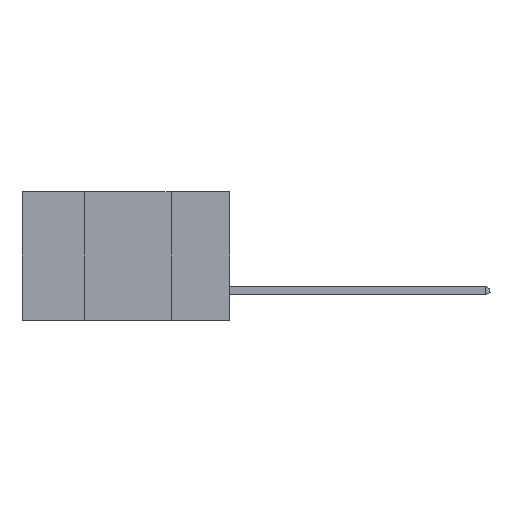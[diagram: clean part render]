
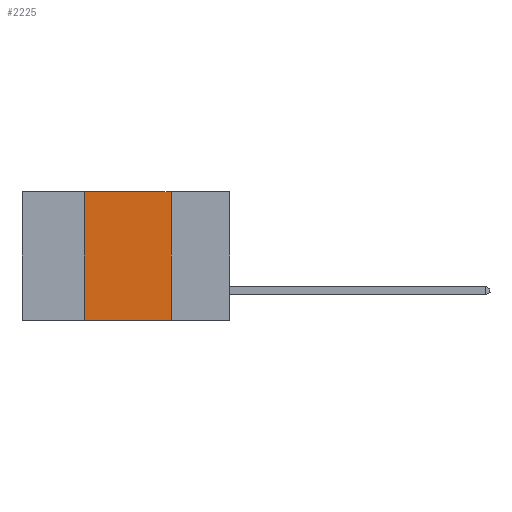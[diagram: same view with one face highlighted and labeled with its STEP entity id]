
A CAD part, left-side view. The second image highlights one B-rep face of the part: STEP entity #2225.
In plain terms, the highlighted planar face has unit normal (-1, 0, 0).
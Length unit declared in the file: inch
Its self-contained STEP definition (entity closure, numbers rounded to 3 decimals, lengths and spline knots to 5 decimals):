
#835 = CARTESIAN_POINT ( 'NONE',  ( 0., 0.42, 0. ) ) ;
#1615 = CARTESIAN_POINT ( 'NONE',  ( 0., 0.6, 0. ) ) ;
#1651 = LINE ( 'NONE', #11527, #7905 ) ;
#1661 = LINE ( 'NONE', #12999, #6748 ) ;
#2039 = VERTEX_POINT ( 'NONE', #8197 ) ;
#2225 = ADVANCED_FACE ( 'NONE', ( #7713 ), #2505, .F. ) ;
#2505 = PLANE ( 'NONE',  #9257 ) ;
#3366 = CARTESIAN_POINT ( 'NONE',  ( 0., 0.17, -0.37 ) ) ;
#3452 = DIRECTION ( 'NONE',  ( 1., 0., 0. ) ) ;
#3993 = ORIENTED_EDGE ( 'NONE', *, *, #11848, .F. ) ;
#5154 = EDGE_LOOP ( 'NONE', ( #3993, #12280, #7296, #12956 ) ) ;
#6724 = CARTESIAN_POINT ( 'NONE',  ( 0., 0.17, 0. ) ) ;
#6748 = VECTOR ( 'NONE', #8850, 39.37008 ) ;
#6766 = DIRECTION ( 'NONE',  ( 0., 0., -1. ) ) ;
#7109 = VECTOR ( 'NONE', #6766, 39.37008 ) ;
#7282 = CARTESIAN_POINT ( 'NONE',  ( 0., 0.42, -0.37 ) ) ;
#7296 = ORIENTED_EDGE ( 'NONE', *, *, #12769, .F. ) ;
#7509 = VERTEX_POINT ( 'NONE', #835 ) ;
#7713 = FACE_OUTER_BOUND ( 'NONE', #5154, .T. ) ;
#7905 = VECTOR ( 'NONE', #8703, 39.37008 ) ;
#8197 = CARTESIAN_POINT ( 'NONE',  ( 0., 0.17, 0. ) ) ;
#8703 = DIRECTION ( 'NONE',  ( 0., 0., 1. ) ) ;
#8850 = DIRECTION ( 'NONE',  ( 0., -1., 0. ) ) ;
#8993 = DIRECTION ( 'NONE',  ( 0., -1., 0. ) ) ;
#9257 = AXIS2_PLACEMENT_3D ( 'NONE', #10899, #3452, #12920 ) ;
#9926 = LINE ( 'NONE', #6724, #7109 ) ;
#10238 = VECTOR ( 'NONE', #8993, 39.37008 ) ;
#10899 = CARTESIAN_POINT ( 'NONE',  ( 0., 0.6, 0. ) ) ;
#11527 = CARTESIAN_POINT ( 'NONE',  ( 0., 0.42, 0. ) ) ;
#11848 = EDGE_CURVE ( 'NONE', #2039, #13370, #9926, .T. ) ;
#12088 = EDGE_CURVE ( 'NONE', #7509, #2039, #13489, .T. ) ;
#12280 = ORIENTED_EDGE ( 'NONE', *, *, #12088, .F. ) ;
#12378 = VERTEX_POINT ( 'NONE', #7282 ) ;
#12567 = EDGE_CURVE ( 'NONE', #12378, #13370, #1661, .T. ) ;
#12769 = EDGE_CURVE ( 'NONE', #12378, #7509, #1651, .T. ) ;
#12920 = DIRECTION ( 'NONE',  ( 0., 0., -1. ) ) ;
#12956 = ORIENTED_EDGE ( 'NONE', *, *, #12567, .T. ) ;
#12999 = CARTESIAN_POINT ( 'NONE',  ( 0., 0.6, -0.37 ) ) ;
#13370 = VERTEX_POINT ( 'NONE', #3366 ) ;
#13489 = LINE ( 'NONE', #1615, #10238 ) ;
